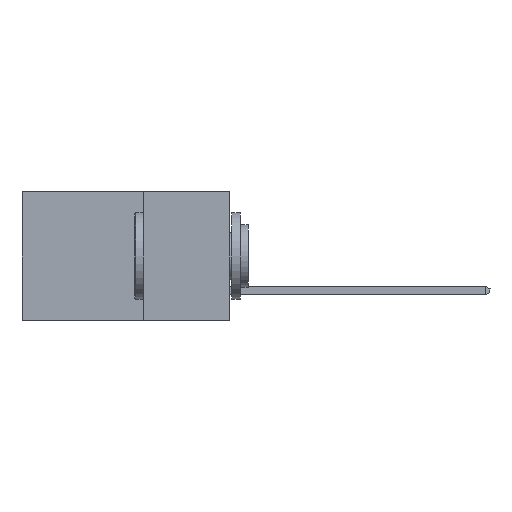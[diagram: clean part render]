
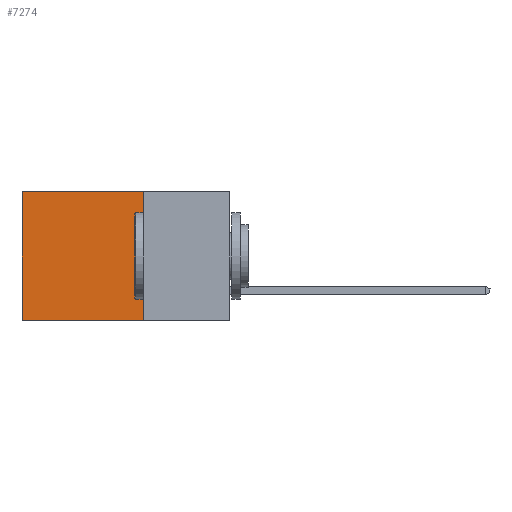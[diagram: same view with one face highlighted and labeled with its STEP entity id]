
A CAD part, left-side view. The second image highlights one B-rep face of the part: STEP entity #7274.
In plain terms, the highlighted planar face has unit normal (-1, 0, 0).
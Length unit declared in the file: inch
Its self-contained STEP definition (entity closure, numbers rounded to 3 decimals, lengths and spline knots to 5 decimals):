
#849 = DIRECTION ( 'NONE',  ( 0., 0., -1. ) ) ;
#1467 = DIRECTION ( 'NONE',  ( 0., 1., 0. ) ) ;
#1798 = CARTESIAN_POINT ( 'NONE',  ( 0.2615, 0.6, -0.37 ) ) ;
#2546 = VERTEX_POINT ( 'NONE', #1798 ) ;
#2610 = ORIENTED_EDGE ( 'NONE', *, *, #12273, .F. ) ;
#2957 = CARTESIAN_POINT ( 'NONE',  ( 0.2615, 0.25, -0.37 ) ) ;
#4570 = EDGE_LOOP ( 'NONE', ( #21780, #2610, #15349, #24181 ) ) ;
#4874 = LINE ( 'NONE', #8899, #14258 ) ;
#5806 = CARTESIAN_POINT ( 'NONE',  ( 0.2615, 0.25, 0. ) ) ;
#6974 = EDGE_CURVE ( 'NONE', #11428, #16613, #20311, .T. ) ;
#7274 = ADVANCED_FACE ( 'NONE', ( #8512 ), #18352, .F. ) ;
#8512 = FACE_OUTER_BOUND ( 'NONE', #4570, .T. ) ;
#8899 = CARTESIAN_POINT ( 'NONE',  ( 0.2615, 0.25, -0.37 ) ) ;
#10492 = CARTESIAN_POINT ( 'NONE',  ( 0.2615, 0.25, 0. ) ) ;
#11296 = LINE ( 'NONE', #24779, #21851 ) ;
#11428 = VERTEX_POINT ( 'NONE', #5806 ) ;
#12273 = EDGE_CURVE ( 'NONE', #18728, #2546, #11296, .T. ) ;
#12645 = AXIS2_PLACEMENT_3D ( 'NONE', #2957, #22375, #18227 ) ;
#13157 = CARTESIAN_POINT ( 'NONE',  ( 0.2615, 0.6, -0.37 ) ) ;
#14258 = VECTOR ( 'NONE', #849, 39.37008 ) ;
#15170 = DIRECTION ( 'NONE',  ( 0., 0., -1. ) ) ;
#15349 = ORIENTED_EDGE ( 'NONE', *, *, #18219, .F. ) ;
#16613 = VERTEX_POINT ( 'NONE', #24869 ) ;
#18219 = EDGE_CURVE ( 'NONE', #11428, #18728, #4874, .T. ) ;
#18227 = DIRECTION ( 'NONE',  ( 0., 0., -1. ) ) ;
#18352 = PLANE ( 'NONE',  #12645 ) ;
#18432 = DIRECTION ( 'NONE',  ( 0., 1., 0. ) ) ;
#18465 = CARTESIAN_POINT ( 'NONE',  ( 0.2615, 0.25, -0.37 ) ) ;
#18728 = VERTEX_POINT ( 'NONE', #18465 ) ;
#20311 = LINE ( 'NONE', #10492, #20729 ) ;
#20729 = VECTOR ( 'NONE', #18432, 39.37008 ) ;
#20768 = VECTOR ( 'NONE', #15170, 39.37008 ) ;
#20804 = EDGE_CURVE ( 'NONE', #16613, #2546, #22486, .T. ) ;
#21780 = ORIENTED_EDGE ( 'NONE', *, *, #20804, .T. ) ;
#21851 = VECTOR ( 'NONE', #1467, 39.37008 ) ;
#22375 = DIRECTION ( 'NONE',  ( 1., 0., 0. ) ) ;
#22486 = LINE ( 'NONE', #13157, #20768 ) ;
#24181 = ORIENTED_EDGE ( 'NONE', *, *, #6974, .T. ) ;
#24779 = CARTESIAN_POINT ( 'NONE',  ( 0.2615, 0.25, -0.37 ) ) ;
#24869 = CARTESIAN_POINT ( 'NONE',  ( 0.2615, 0.6, 0. ) ) ;
